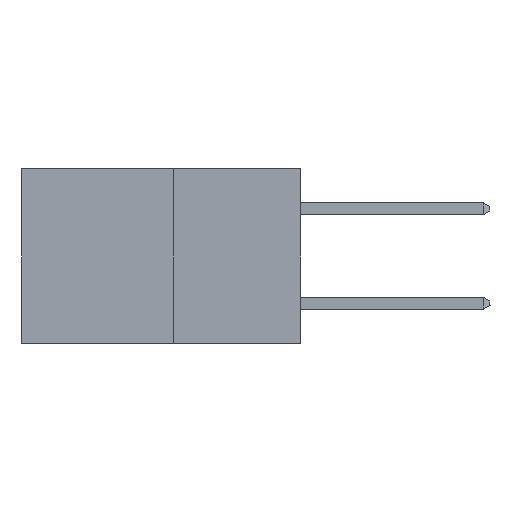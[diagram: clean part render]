
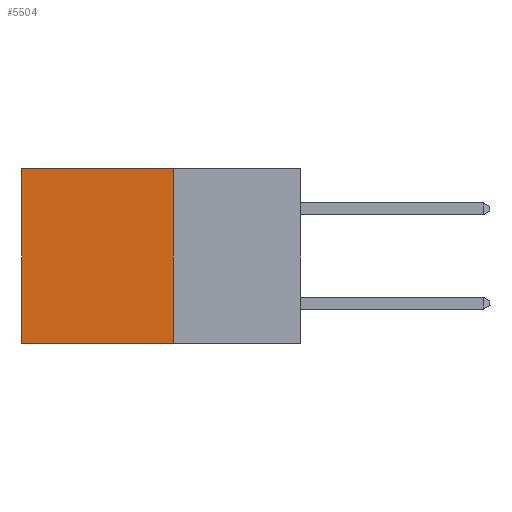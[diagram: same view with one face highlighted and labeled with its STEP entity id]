
A CAD part, left-side view. The second image highlights one B-rep face of the part: STEP entity #5504.
In plain terms, the highlighted planar face has unit normal (-1, 0, 0).
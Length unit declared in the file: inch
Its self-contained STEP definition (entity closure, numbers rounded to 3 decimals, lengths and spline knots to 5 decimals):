
#494 = PLANE ( 'NONE',  #1728 ) ;
#1526 = FACE_OUTER_BOUND ( 'NONE', #14370, .T. ) ;
#1728 = AXIS2_PLACEMENT_3D ( 'NONE', #15942, #6316, #19824 ) ;
#2794 = CARTESIAN_POINT ( 'NONE',  ( 0.277, 0.59, -0.37 ) ) ;
#2854 = VECTOR ( 'NONE', #23966, 39.37008 ) ;
#3744 = EDGE_CURVE ( 'NONE', #24323, #22511, #23364, .T. ) ;
#4670 = VECTOR ( 'NONE', #8462, 39.37008 ) ;
#4764 = ORIENTED_EDGE ( 'NONE', *, *, #8100, .F. ) ;
#5290 = VERTEX_POINT ( 'NONE', #9376 ) ;
#5504 = ADVANCED_FACE ( 'NONE', ( #1526 ), #494, .F. ) ;
#6316 = DIRECTION ( 'NONE',  ( 1., 0., 0. ) ) ;
#7899 = ORIENTED_EDGE ( 'NONE', *, *, #23299, .T. ) ;
#8100 = EDGE_CURVE ( 'NONE', #23194, #22511, #13669, .T. ) ;
#8462 = DIRECTION ( 'NONE',  ( 0., 1., 0. ) ) ;
#9281 = VECTOR ( 'NONE', #19375, 39.37008 ) ;
#9376 = CARTESIAN_POINT ( 'NONE',  ( 0.277, 0.27, 0. ) ) ;
#11618 = CARTESIAN_POINT ( 'NONE',  ( 0.277, 0.59, -0.37 ) ) ;
#12793 = VECTOR ( 'NONE', #16490, 39.37008 ) ;
#13669 = LINE ( 'NONE', #20041, #4670 ) ;
#14370 = EDGE_LOOP ( 'NONE', ( #17477, #4764, #20823, #7899 ) ) ;
#14536 = CARTESIAN_POINT ( 'NONE',  ( 0.277, 0.27, -0.37 ) ) ;
#15942 = CARTESIAN_POINT ( 'NONE',  ( 0.277, 0.27, -0.37 ) ) ;
#16490 = DIRECTION ( 'NONE',  ( 0., 0., -1. ) ) ;
#17431 = CARTESIAN_POINT ( 'NONE',  ( 0.277, 0.27, 0. ) ) ;
#17477 = ORIENTED_EDGE ( 'NONE', *, *, #3744, .T. ) ;
#19081 = EDGE_CURVE ( 'NONE', #5290, #23194, #23073, .T. ) ;
#19138 = CARTESIAN_POINT ( 'NONE',  ( 0.277, 0.59, 0. ) ) ;
#19375 = DIRECTION ( 'NONE',  ( 0., 1., 0. ) ) ;
#19824 = DIRECTION ( 'NONE',  ( 0., 0., -1. ) ) ;
#20041 = CARTESIAN_POINT ( 'NONE',  ( 0.277, 0.27, -0.37 ) ) ;
#20823 = ORIENTED_EDGE ( 'NONE', *, *, #19081, .F. ) ;
#22511 = VERTEX_POINT ( 'NONE', #11618 ) ;
#23073 = LINE ( 'NONE', #14536, #12793 ) ;
#23194 = VERTEX_POINT ( 'NONE', #24946 ) ;
#23299 = EDGE_CURVE ( 'NONE', #5290, #24323, #24716, .T. ) ;
#23364 = LINE ( 'NONE', #2794, #2854 ) ;
#23966 = DIRECTION ( 'NONE',  ( 0., 0., -1. ) ) ;
#24323 = VERTEX_POINT ( 'NONE', #19138 ) ;
#24716 = LINE ( 'NONE', #17431, #9281 ) ;
#24946 = CARTESIAN_POINT ( 'NONE',  ( 0.277, 0.27, -0.37 ) ) ;
